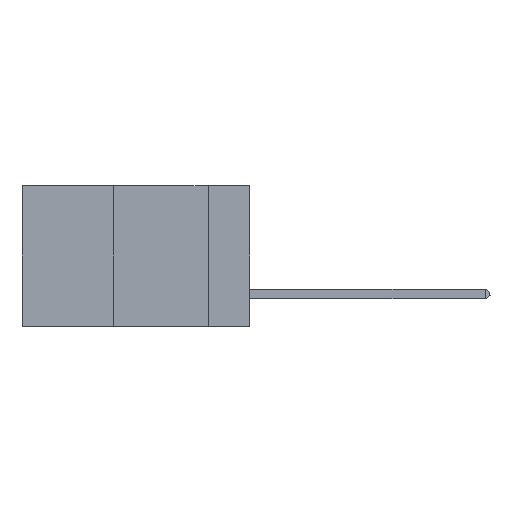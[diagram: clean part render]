
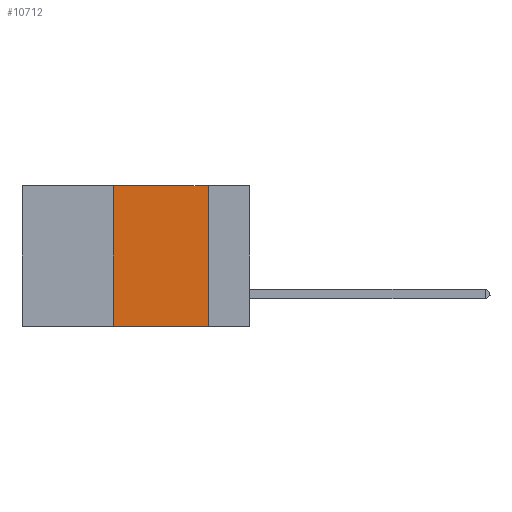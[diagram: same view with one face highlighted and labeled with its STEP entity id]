
A CAD part, left-side view. The second image highlights one B-rep face of the part: STEP entity #10712.
In plain terms, the highlighted planar face has unit normal (-1, 0, 0).
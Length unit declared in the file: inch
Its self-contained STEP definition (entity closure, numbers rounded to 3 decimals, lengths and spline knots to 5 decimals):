
#1020 = VERTEX_POINT ( 'NONE', #4804 ) ;
#1028 = CARTESIAN_POINT ( 'NONE',  ( 0., 0.36, -0.37 ) ) ;
#1210 = ORIENTED_EDGE ( 'NONE', *, *, #1732, .T. ) ;
#1239 = CARTESIAN_POINT ( 'NONE',  ( 0., 0.6, 0. ) ) ;
#1732 = EDGE_CURVE ( 'NONE', #5163, #1020, #2513, .T. ) ;
#1844 = ORIENTED_EDGE ( 'NONE', *, *, #16039, .F. ) ;
#1951 = CARTESIAN_POINT ( 'NONE',  ( 0., 0.36, 0. ) ) ;
#2337 = VERTEX_POINT ( 'NONE', #11074 ) ;
#2349 = DIRECTION ( 'NONE',  ( 0., 0., -1. ) ) ;
#2513 = LINE ( 'NONE', #13834, #5440 ) ;
#3161 = DIRECTION ( 'NONE',  ( 0., 0., -1. ) ) ;
#4139 = EDGE_CURVE ( 'NONE', #5163, #2337, #8046, .T. ) ;
#4234 = ORIENTED_EDGE ( 'NONE', *, *, #10497, .F. ) ;
#4804 = CARTESIAN_POINT ( 'NONE',  ( 0., 0.11, -0.37 ) ) ;
#4961 = DIRECTION ( 'NONE',  ( 0., -1., 0. ) ) ;
#5035 = PLANE ( 'NONE',  #5254 ) ;
#5163 = VERTEX_POINT ( 'NONE', #1028 ) ;
#5254 = AXIS2_PLACEMENT_3D ( 'NONE', #1239, #7561, #2349 ) ;
#5440 = VECTOR ( 'NONE', #13670, 39.37008 ) ;
#5615 = LINE ( 'NONE', #9779, #15431 ) ;
#5695 = CARTESIAN_POINT ( 'NONE',  ( 0., 0.11, 0. ) ) ;
#6103 = EDGE_LOOP ( 'NONE', ( #4234, #1844, #12785, #1210 ) ) ;
#6338 = VECTOR ( 'NONE', #3161, 39.37008 ) ;
#7104 = FACE_OUTER_BOUND ( 'NONE', #6103, .T. ) ;
#7125 = LINE ( 'NONE', #5695, #6338 ) ;
#7468 = VECTOR ( 'NONE', #10717, 39.37008 ) ;
#7561 = DIRECTION ( 'NONE',  ( 1., 0., 0. ) ) ;
#8046 = LINE ( 'NONE', #1951, #7468 ) ;
#9779 = CARTESIAN_POINT ( 'NONE',  ( 0., 0.6, 0. ) ) ;
#10497 = EDGE_CURVE ( 'NONE', #10880, #1020, #7125, .T. ) ;
#10712 = ADVANCED_FACE ( 'NONE', ( #7104 ), #5035, .F. ) ;
#10717 = DIRECTION ( 'NONE',  ( 0., 0., 1. ) ) ;
#10880 = VERTEX_POINT ( 'NONE', #15294 ) ;
#11074 = CARTESIAN_POINT ( 'NONE',  ( 0., 0.36, 0. ) ) ;
#12785 = ORIENTED_EDGE ( 'NONE', *, *, #4139, .F. ) ;
#13670 = DIRECTION ( 'NONE',  ( 0., -1., 0. ) ) ;
#13834 = CARTESIAN_POINT ( 'NONE',  ( 0., 0.6, -0.37 ) ) ;
#15294 = CARTESIAN_POINT ( 'NONE',  ( 0., 0.11, 0. ) ) ;
#15431 = VECTOR ( 'NONE', #4961, 39.37008 ) ;
#16039 = EDGE_CURVE ( 'NONE', #2337, #10880, #5615, .T. ) ;
